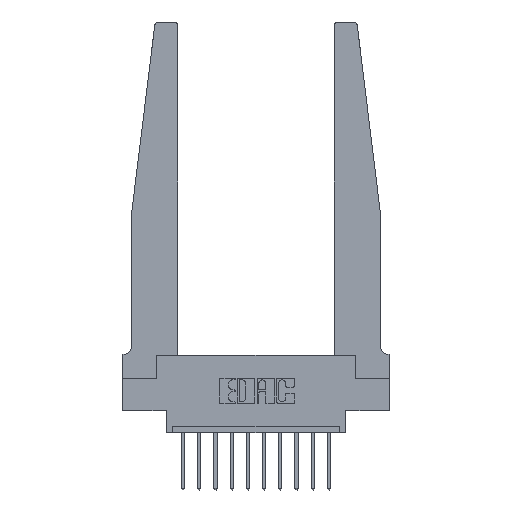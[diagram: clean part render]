
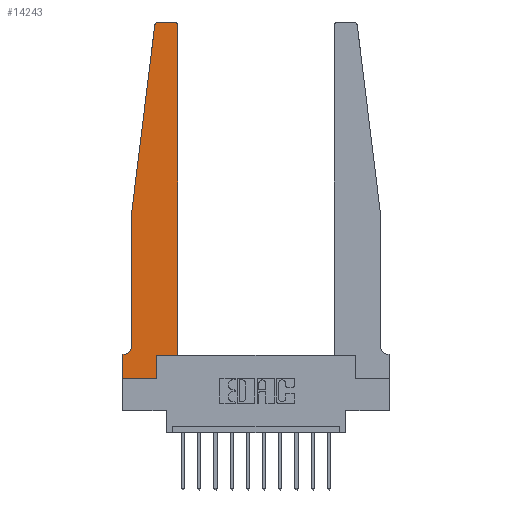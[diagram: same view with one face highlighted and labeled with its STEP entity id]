
A CAD part, top view. The second image highlights one B-rep face of the part: STEP entity #14243.
In plain terms, the highlighted planar face has unit normal (0, 0, 1).
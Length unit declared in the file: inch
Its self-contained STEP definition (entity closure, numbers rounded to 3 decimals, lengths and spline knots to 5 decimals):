
#23 = CARTESIAN_POINT ( 'NONE',  ( 0.065, 0.1875, 0.37 ) ) ;
#79 = VECTOR ( 'NONE', #14712, 39.37008 ) ;
#113 = CARTESIAN_POINT ( 'NONE',  ( 0.425, 0.18, 0.37 ) ) ;
#264 = VECTOR ( 'NONE', #9320, 39.37008 ) ;
#482 = DIRECTION ( 'NONE',  ( 0., 1., 0. ) ) ;
#527 = ORIENTED_EDGE ( 'NONE', *, *, #2443, .T. ) ;
#574 = EDGE_CURVE ( 'NONE', #11823, #10328, #11015, .T. ) ;
#690 = CARTESIAN_POINT ( 'NONE',  ( 0.425, 0.18, 0.37 ) ) ;
#803 = CARTESIAN_POINT ( 'NONE',  ( 0.015, 0.2375, 0.37 ) ) ;
#806 = EDGE_CURVE ( 'NONE', #1027, #1579, #4580, .T. ) ;
#1027 = VERTEX_POINT ( 'NONE', #9207 ) ;
#1240 = DIRECTION ( 'NONE',  ( 0., -1., 0. ) ) ;
#1297 = CARTESIAN_POINT ( 'NONE',  ( 0., 0.1875, 0.37 ) ) ;
#1485 = DIRECTION ( 'NONE',  ( 1., 0., 0. ) ) ;
#1579 = VERTEX_POINT ( 'NONE', #14408 ) ;
#1588 = DIRECTION ( 'NONE',  ( 0., -1., 0. ) ) ;
#1787 = VERTEX_POINT ( 'NONE', #7739 ) ;
#1799 = EDGE_CURVE ( 'NONE', #15135, #6949, #15558, .T. ) ;
#2443 = EDGE_CURVE ( 'NONE', #8825, #7960, #8415, .T. ) ;
#3088 = DIRECTION ( 'NONE',  ( 1., 0., 0. ) ) ;
#3218 = CARTESIAN_POINT ( 'NONE',  ( 0.065, 1.25, 0.37 ) ) ;
#3276 = CARTESIAN_POINT ( 'NONE',  ( 0.27653, 2.72, 0.37 ) ) ;
#3682 = DIRECTION ( 'NONE',  ( -0.122, -0.992, 0. ) ) ;
#4158 = AXIS2_PLACEMENT_3D ( 'NONE', #803, #4388, #12988 ) ;
#4219 = CARTESIAN_POINT ( 'NONE',  ( 0.015, 0.1875, 0.37 ) ) ;
#4296 = EDGE_CURVE ( 'NONE', #7960, #11286, #14547, .T. ) ;
#4388 = DIRECTION ( 'NONE',  ( 0., 0., -1. ) ) ;
#4580 = LINE ( 'NONE', #11802, #13172 ) ;
#4712 = AXIS2_PLACEMENT_3D ( 'NONE', #6186, #11316, #12284 ) ;
#4724 = VECTOR ( 'NONE', #1588, 39.37008 ) ;
#4748 = LINE ( 'NONE', #11984, #10725 ) ;
#4999 = EDGE_CURVE ( 'NONE', #1787, #11823, #13233, .T. ) ;
#5081 = ORIENTED_EDGE ( 'NONE', *, *, #1799, .T. ) ;
#6029 = CARTESIAN_POINT ( 'NONE',  ( 0., 0., 0.37 ) ) ;
#6186 = CARTESIAN_POINT ( 'NONE',  ( 0., 0.1875, 0.37 ) ) ;
#6348 = ORIENTED_EDGE ( 'NONE', *, *, #12522, .T. ) ;
#6559 = LINE ( 'NONE', #11458, #7248 ) ;
#6637 = ORIENTED_EDGE ( 'NONE', *, *, #4999, .T. ) ;
#6774 = ORIENTED_EDGE ( 'NONE', *, *, #4296, .T. ) ;
#6887 = AXIS2_PLACEMENT_3D ( 'NONE', #3276, #9306, #14217 ) ;
#6949 = VERTEX_POINT ( 'NONE', #12393 ) ;
#7039 = VERTEX_POINT ( 'NONE', #690 ) ;
#7248 = VECTOR ( 'NONE', #482, 39.37008 ) ;
#7491 = CARTESIAN_POINT ( 'NONE',  ( 0.395, 2.72, 0.37 ) ) ;
#7561 = PLANE ( 'NONE',  #4712 ) ;
#7676 = LINE ( 'NONE', #9982, #4724 ) ;
#7739 = CARTESIAN_POINT ( 'NONE',  ( 0.065, 0.2375, 0.37 ) ) ;
#7757 = VECTOR ( 'NONE', #12237, 39.37008 ) ;
#7960 = VERTEX_POINT ( 'NONE', #15782 ) ;
#8259 = EDGE_CURVE ( 'NONE', #1579, #7039, #15851, .T. ) ;
#8415 = CIRCLE ( 'NONE', #6887, 0.03 ) ;
#8653 = EDGE_CURVE ( 'NONE', #11286, #1787, #4748, .T. ) ;
#8737 = ORIENTED_EDGE ( 'NONE', *, *, #806, .T. ) ;
#8825 = VERTEX_POINT ( 'NONE', #8842 ) ;
#8838 = FACE_OUTER_BOUND ( 'NONE', #10349, .T. ) ;
#8842 = CARTESIAN_POINT ( 'NONE',  ( 0.27653, 2.75, 0.37 ) ) ;
#9195 = ORIENTED_EDGE ( 'NONE', *, *, #13244, .T. ) ;
#9207 = CARTESIAN_POINT ( 'NONE',  ( 0.2605, 0., 0.37 ) ) ;
#9306 = DIRECTION ( 'NONE',  ( 0., 0., 1. ) ) ;
#9320 = DIRECTION ( 'NONE',  ( -1., 0., 0. ) ) ;
#9859 = ORIENTED_EDGE ( 'NONE', *, *, #8653, .T. ) ;
#9891 = AXIS2_PLACEMENT_3D ( 'NONE', #7491, #12469, #1485 ) ;
#9982 = CARTESIAN_POINT ( 'NONE',  ( 0., 0., 0.37 ) ) ;
#10306 = EDGE_CURVE ( 'NONE', #6949, #8825, #13013, .T. ) ;
#10328 = VERTEX_POINT ( 'NONE', #1297 ) ;
#10349 = EDGE_LOOP ( 'NONE', ( #14675, #527, #6774, #9859, #6637, #13334, #11375, #6348, #8737, #12822, #9195, #5081 ) ) ;
#10725 = VECTOR ( 'NONE', #1240, 39.37008 ) ;
#10829 = VECTOR ( 'NONE', #3088, 39.37008 ) ;
#11015 = LINE ( 'NONE', #23, #79 ) ;
#11056 = VECTOR ( 'NONE', #3682, 39.37008 ) ;
#11286 = VERTEX_POINT ( 'NONE', #3218 ) ;
#11316 = DIRECTION ( 'NONE',  ( 0., 0., 1. ) ) ;
#11375 = ORIENTED_EDGE ( 'NONE', *, *, #14810, .T. ) ;
#11458 = CARTESIAN_POINT ( 'NONE',  ( 0.425, 0.18, 0.37 ) ) ;
#11802 = CARTESIAN_POINT ( 'NONE',  ( 0.2605, 0.18, 0.37 ) ) ;
#11823 = VERTEX_POINT ( 'NONE', #4219 ) ;
#11984 = CARTESIAN_POINT ( 'NONE',  ( 0.065, 1.25, 0.37 ) ) ;
#12130 = CARTESIAN_POINT ( 'NONE',  ( 0.065, 1.25, 0.37 ) ) ;
#12237 = DIRECTION ( 'NONE',  ( 1., 0., 0. ) ) ;
#12284 = DIRECTION ( 'NONE',  ( 1., 0., 0. ) ) ;
#12393 = CARTESIAN_POINT ( 'NONE',  ( 0.395, 2.75, 0.37 ) ) ;
#12469 = DIRECTION ( 'NONE',  ( 0., 0., 1. ) ) ;
#12522 = EDGE_CURVE ( 'NONE', #15326, #1027, #14020, .T. ) ;
#12822 = ORIENTED_EDGE ( 'NONE', *, *, #8259, .T. ) ;
#12988 = DIRECTION ( 'NONE',  ( -1., 0., 0. ) ) ;
#13013 = LINE ( 'NONE', #14000, #264 ) ;
#13172 = VECTOR ( 'NONE', #13548, 39.37008 ) ;
#13233 = CIRCLE ( 'NONE', #4158, 0.05 ) ;
#13244 = EDGE_CURVE ( 'NONE', #7039, #15135, #6559, .T. ) ;
#13334 = ORIENTED_EDGE ( 'NONE', *, *, #574, .T. ) ;
#13548 = DIRECTION ( 'NONE',  ( 0., 1., 0. ) ) ;
#14000 = CARTESIAN_POINT ( 'NONE',  ( 0.25, 2.75, 0.37 ) ) ;
#14020 = LINE ( 'NONE', #14095, #10829 ) ;
#14095 = CARTESIAN_POINT ( 'NONE',  ( 0., 0., 0.37 ) ) ;
#14217 = DIRECTION ( 'NONE',  ( 1., 0., 0. ) ) ;
#14243 = ADVANCED_FACE ( 'NONE', ( #8838 ), #7561, .T. ) ;
#14408 = CARTESIAN_POINT ( 'NONE',  ( 0.2605, 0.18, 0.37 ) ) ;
#14547 = LINE ( 'NONE', #12130, #11056 ) ;
#14675 = ORIENTED_EDGE ( 'NONE', *, *, #10306, .T. ) ;
#14712 = DIRECTION ( 'NONE',  ( -1., 0., 0. ) ) ;
#14810 = EDGE_CURVE ( 'NONE', #10328, #15326, #7676, .T. ) ;
#15038 = CARTESIAN_POINT ( 'NONE',  ( 0.425, 2.72, 0.37 ) ) ;
#15135 = VERTEX_POINT ( 'NONE', #15038 ) ;
#15326 = VERTEX_POINT ( 'NONE', #6029 ) ;
#15558 = CIRCLE ( 'NONE', #9891, 0.03 ) ;
#15782 = CARTESIAN_POINT ( 'NONE',  ( 0.24675, 2.72367, 0.37 ) ) ;
#15851 = LINE ( 'NONE', #113, #7757 ) ;
